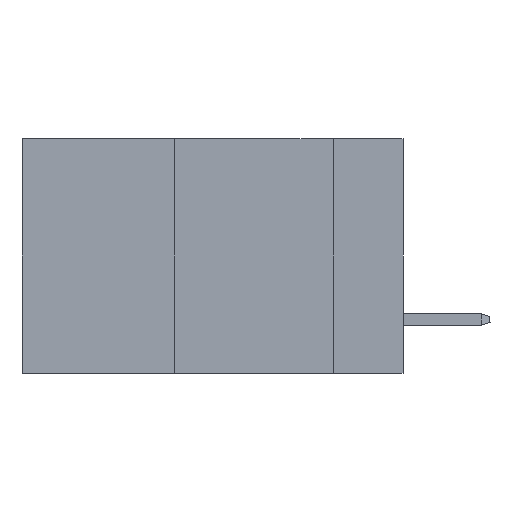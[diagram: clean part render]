
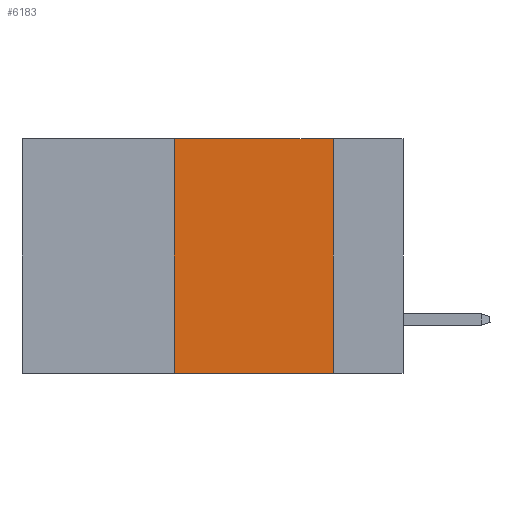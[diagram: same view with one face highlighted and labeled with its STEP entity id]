
A CAD part, left-side view. The second image highlights one B-rep face of the part: STEP entity #6183.
In plain terms, the highlighted planar face has unit normal (-1, 0, 0).
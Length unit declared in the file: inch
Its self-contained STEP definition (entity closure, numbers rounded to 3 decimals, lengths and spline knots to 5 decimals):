
#452 = VECTOR ( 'NONE', #16745, 39.37008 ) ;
#1067 = DIRECTION ( 'NONE',  ( 0., 0., -1. ) ) ;
#1375 = VECTOR ( 'NONE', #3356, 39.37008 ) ;
#1976 = CARTESIAN_POINT ( 'NONE',  ( 0., 0.6, -0.37 ) ) ;
#2244 = VECTOR ( 'NONE', #15831, 39.37008 ) ;
#2732 = CARTESIAN_POINT ( 'NONE',  ( 0., 0.36, -0.37 ) ) ;
#3150 = ORIENTED_EDGE ( 'NONE', *, *, #14498, .F. ) ;
#3356 = DIRECTION ( 'NONE',  ( 0., -1., 0. ) ) ;
#3402 = LINE ( 'NONE', #1976, #452 ) ;
#5460 = CARTESIAN_POINT ( 'NONE',  ( 0., 0.36, 0. ) ) ;
#6183 = ADVANCED_FACE ( 'NONE', ( #7738 ), #17251, .F. ) ;
#7154 = VERTEX_POINT ( 'NONE', #7962 ) ;
#7597 = EDGE_CURVE ( 'NONE', #15620, #9812, #17389, .T. ) ;
#7665 = VERTEX_POINT ( 'NONE', #14832 ) ;
#7738 = FACE_OUTER_BOUND ( 'NONE', #15710, .T. ) ;
#7962 = CARTESIAN_POINT ( 'NONE',  ( 0., 0.11, 0. ) ) ;
#9812 = VERTEX_POINT ( 'NONE', #5460 ) ;
#9846 = EDGE_CURVE ( 'NONE', #15620, #7665, #3402, .T. ) ;
#10024 = LINE ( 'NONE', #12510, #1375 ) ;
#11651 = DIRECTION ( 'NONE',  ( 0., 0., -1. ) ) ;
#11881 = CARTESIAN_POINT ( 'NONE',  ( 0., 0.36, 0. ) ) ;
#12510 = CARTESIAN_POINT ( 'NONE',  ( 0., 0.6, 0. ) ) ;
#12676 = AXIS2_PLACEMENT_3D ( 'NONE', #14576, #14422, #11651 ) ;
#13039 = ORIENTED_EDGE ( 'NONE', *, *, #14943, .F. ) ;
#13158 = CARTESIAN_POINT ( 'NONE',  ( 0., 0.11, 0. ) ) ;
#14422 = DIRECTION ( 'NONE',  ( 1., 0., 0. ) ) ;
#14498 = EDGE_CURVE ( 'NONE', #9812, #7154, #10024, .T. ) ;
#14576 = CARTESIAN_POINT ( 'NONE',  ( 0., 0.6, 0. ) ) ;
#14832 = CARTESIAN_POINT ( 'NONE',  ( 0., 0.11, -0.37 ) ) ;
#14943 = EDGE_CURVE ( 'NONE', #7154, #7665, #15854, .T. ) ;
#15620 = VERTEX_POINT ( 'NONE', #2732 ) ;
#15710 = EDGE_LOOP ( 'NONE', ( #13039, #3150, #17113, #15946 ) ) ;
#15831 = DIRECTION ( 'NONE',  ( 0., 0., 1. ) ) ;
#15854 = LINE ( 'NONE', #13158, #15890 ) ;
#15890 = VECTOR ( 'NONE', #1067, 39.37008 ) ;
#15946 = ORIENTED_EDGE ( 'NONE', *, *, #9846, .T. ) ;
#16745 = DIRECTION ( 'NONE',  ( 0., -1., 0. ) ) ;
#17113 = ORIENTED_EDGE ( 'NONE', *, *, #7597, .F. ) ;
#17251 = PLANE ( 'NONE',  #12676 ) ;
#17389 = LINE ( 'NONE', #11881, #2244 ) ;
